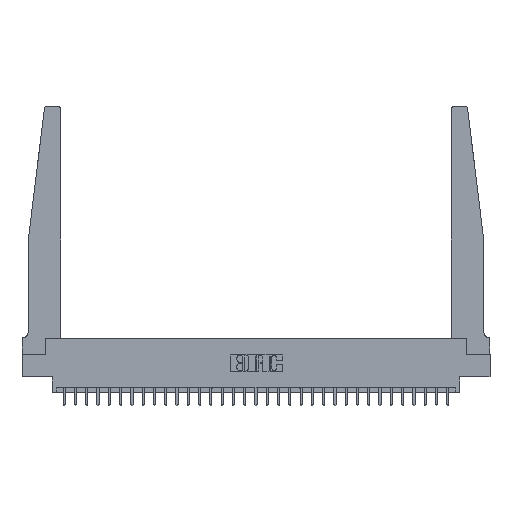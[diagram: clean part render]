
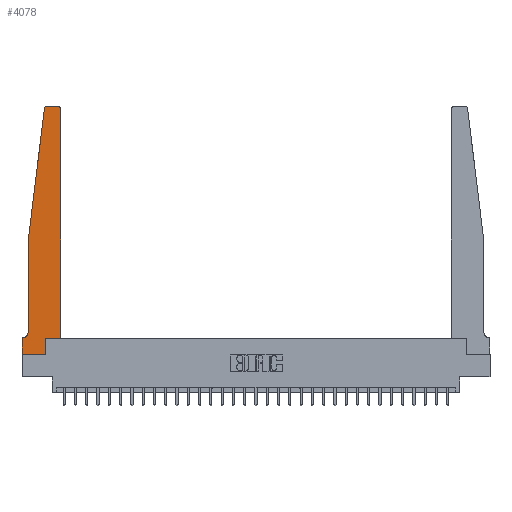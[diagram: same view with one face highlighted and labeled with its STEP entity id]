
A CAD part, top view. The second image highlights one B-rep face of the part: STEP entity #4078.
In plain terms, the highlighted planar face has unit normal (0, 0, 1).
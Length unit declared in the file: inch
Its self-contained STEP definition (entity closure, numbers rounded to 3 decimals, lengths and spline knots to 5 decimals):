
#764 = CARTESIAN_POINT ( 'NONE',  ( 0.27653, 2.75, 0.37 ) ) ;
#829 = FACE_OUTER_BOUND ( 'NONE', #19443, .T. ) ;
#895 = VERTEX_POINT ( 'NONE', #12179 ) ;
#1445 = ORIENTED_EDGE ( 'NONE', *, *, #22652, .T. ) ;
#1629 = ORIENTED_EDGE ( 'NONE', *, *, #19294, .T. ) ;
#1719 = ORIENTED_EDGE ( 'NONE', *, *, #20639, .T. ) ;
#1783 = EDGE_CURVE ( 'NONE', #9734, #4977, #10332, .T. ) ;
#1935 = CARTESIAN_POINT ( 'NONE',  ( 0.425, 2.72, 0.37 ) ) ;
#2194 = ORIENTED_EDGE ( 'NONE', *, *, #1783, .T. ) ;
#2510 = EDGE_CURVE ( 'NONE', #13632, #2628, #15795, .T. ) ;
#2628 = VERTEX_POINT ( 'NONE', #12297 ) ;
#3039 = PLANE ( 'NONE',  #23411 ) ;
#4078 = ADVANCED_FACE ( 'NONE', ( #829 ), #3039, .T. ) ;
#4294 = VERTEX_POINT ( 'NONE', #9382 ) ;
#4536 = CARTESIAN_POINT ( 'NONE',  ( 0.065, 1.25, 0.37 ) ) ;
#4634 = CARTESIAN_POINT ( 'NONE',  ( 0.425, 0.18, 0.37 ) ) ;
#4977 = VERTEX_POINT ( 'NONE', #10796 ) ;
#5024 = VECTOR ( 'NONE', #6549, 39.37008 ) ;
#5592 = VERTEX_POINT ( 'NONE', #13567 ) ;
#5667 = CARTESIAN_POINT ( 'NONE',  ( 0.425, 0.18, 0.37 ) ) ;
#6128 = LINE ( 'NONE', #6573, #9366 ) ;
#6343 = VERTEX_POINT ( 'NONE', #10515 ) ;
#6492 = LINE ( 'NONE', #9685, #26408 ) ;
#6549 = DIRECTION ( 'NONE',  ( -0.122, -0.992, 0. ) ) ;
#6573 = CARTESIAN_POINT ( 'NONE',  ( 0.065, 0.1875, 0.37 ) ) ;
#7783 = DIRECTION ( 'NONE',  ( 0., 0., 1. ) ) ;
#9280 = AXIS2_PLACEMENT_3D ( 'NONE', #16641, #12321, #14843 ) ;
#9366 = VECTOR ( 'NONE', #15596, 39.37008 ) ;
#9382 = CARTESIAN_POINT ( 'NONE',  ( 0.395, 2.75, 0.37 ) ) ;
#9648 = DIRECTION ( 'NONE',  ( 0., 1., 0. ) ) ;
#9685 = CARTESIAN_POINT ( 'NONE',  ( 0., 0., 0.37 ) ) ;
#9734 = VERTEX_POINT ( 'NONE', #24528 ) ;
#10059 = VECTOR ( 'NONE', #18448, 39.37008 ) ;
#10228 = ORIENTED_EDGE ( 'NONE', *, *, #18574, .T. ) ;
#10332 = LINE ( 'NONE', #20980, #11609 ) ;
#10515 = CARTESIAN_POINT ( 'NONE',  ( 0., 0.1875, 0.37 ) ) ;
#10796 = CARTESIAN_POINT ( 'NONE',  ( 0.2605, 0.18, 0.37 ) ) ;
#10844 = DIRECTION ( 'NONE',  ( 0., 0., -1. ) ) ;
#11584 = VECTOR ( 'NONE', #13251, 39.37008 ) ;
#11609 = VECTOR ( 'NONE', #14493, 39.37008 ) ;
#11685 = ORIENTED_EDGE ( 'NONE', *, *, #26746, .T. ) ;
#12131 = EDGE_CURVE ( 'NONE', #2628, #895, #24885, .T. ) ;
#12179 = CARTESIAN_POINT ( 'NONE',  ( 0.015, 0.1875, 0.37 ) ) ;
#12297 = CARTESIAN_POINT ( 'NONE',  ( 0.065, 0.2375, 0.37 ) ) ;
#12321 = DIRECTION ( 'NONE',  ( 0., 0., 1. ) ) ;
#12524 = DIRECTION ( 'NONE',  ( 0., 0., 1. ) ) ;
#12640 = VERTEX_POINT ( 'NONE', #1935 ) ;
#13251 = DIRECTION ( 'NONE',  ( -1., 0., 0. ) ) ;
#13420 = ORIENTED_EDGE ( 'NONE', *, *, #2510, .T. ) ;
#13567 = CARTESIAN_POINT ( 'NONE',  ( 0., 0., 0.37 ) ) ;
#13612 = ORIENTED_EDGE ( 'NONE', *, *, #20744, .T. ) ;
#13632 = VERTEX_POINT ( 'NONE', #26166 ) ;
#13639 = CARTESIAN_POINT ( 'NONE',  ( 0., 0., 0.37 ) ) ;
#13667 = LINE ( 'NONE', #4634, #24082 ) ;
#14493 = DIRECTION ( 'NONE',  ( 0., 1., 0. ) ) ;
#14835 = DIRECTION ( 'NONE',  ( 1., 0., 0. ) ) ;
#14843 = DIRECTION ( 'NONE',  ( 1., 0., 0. ) ) ;
#14905 = CARTESIAN_POINT ( 'NONE',  ( 0.27653, 2.72, 0.37 ) ) ;
#15496 = CARTESIAN_POINT ( 'NONE',  ( 0.25, 2.75, 0.37 ) ) ;
#15596 = DIRECTION ( 'NONE',  ( -1., 0., 0. ) ) ;
#15706 = EDGE_CURVE ( 'NONE', #6343, #5592, #17655, .T. ) ;
#15795 = LINE ( 'NONE', #4536, #10059 ) ;
#16641 = CARTESIAN_POINT ( 'NONE',  ( 0.395, 2.72, 0.37 ) ) ;
#16959 = AXIS2_PLACEMENT_3D ( 'NONE', #14905, #12524, #19343 ) ;
#16987 = ORIENTED_EDGE ( 'NONE', *, *, #23023, .T. ) ;
#17655 = LINE ( 'NONE', #13639, #22836 ) ;
#18322 = AXIS2_PLACEMENT_3D ( 'NONE', #19724, #10844, #21916 ) ;
#18448 = DIRECTION ( 'NONE',  ( 0., -1., 0. ) ) ;
#18574 = EDGE_CURVE ( 'NONE', #4294, #22357, #19912, .T. ) ;
#18887 = DIRECTION ( 'NONE',  ( 1., 0., 0. ) ) ;
#18910 = ORIENTED_EDGE ( 'NONE', *, *, #15706, .T. ) ;
#19155 = VECTOR ( 'NONE', #14835, 39.37008 ) ;
#19294 = EDGE_CURVE ( 'NONE', #4977, #27153, #21480, .T. ) ;
#19343 = DIRECTION ( 'NONE',  ( 1., 0., 0. ) ) ;
#19443 = EDGE_LOOP ( 'NONE', ( #10228, #1445, #13612, #13420, #23301, #16987, #18910, #11685, #2194, #1629, #28162, #1719 ) ) ;
#19724 = CARTESIAN_POINT ( 'NONE',  ( 0.015, 0.2375, 0.37 ) ) ;
#19912 = LINE ( 'NONE', #15496, #11584 ) ;
#20639 = EDGE_CURVE ( 'NONE', #12640, #4294, #23877, .T. ) ;
#20744 = EDGE_CURVE ( 'NONE', #26954, #13632, #21901, .T. ) ;
#20980 = CARTESIAN_POINT ( 'NONE',  ( 0.2605, 0.18, 0.37 ) ) ;
#21480 = LINE ( 'NONE', #5667, #19155 ) ;
#21901 = LINE ( 'NONE', #28800, #5024 ) ;
#21916 = DIRECTION ( 'NONE',  ( -1., 0., 0. ) ) ;
#22357 = VERTEX_POINT ( 'NONE', #764 ) ;
#22627 = DIRECTION ( 'NONE',  ( 0., -1., 0. ) ) ;
#22652 = EDGE_CURVE ( 'NONE', #22357, #26954, #28653, .T. ) ;
#22832 = DIRECTION ( 'NONE',  ( 1., 0., 0. ) ) ;
#22836 = VECTOR ( 'NONE', #22627, 39.37008 ) ;
#23023 = EDGE_CURVE ( 'NONE', #895, #6343, #6128, .T. ) ;
#23115 = EDGE_CURVE ( 'NONE', #27153, #12640, #13667, .T. ) ;
#23301 = ORIENTED_EDGE ( 'NONE', *, *, #12131, .T. ) ;
#23325 = CARTESIAN_POINT ( 'NONE',  ( 0.24675, 2.72367, 0.37 ) ) ;
#23411 = AXIS2_PLACEMENT_3D ( 'NONE', #25498, #7783, #18887 ) ;
#23877 = CIRCLE ( 'NONE', #9280, 0.03 ) ;
#24082 = VECTOR ( 'NONE', #9648, 39.37008 ) ;
#24528 = CARTESIAN_POINT ( 'NONE',  ( 0.2605, 0., 0.37 ) ) ;
#24885 = CIRCLE ( 'NONE', #18322, 0.05 ) ;
#24932 = CARTESIAN_POINT ( 'NONE',  ( 0.425, 0.18, 0.37 ) ) ;
#25498 = CARTESIAN_POINT ( 'NONE',  ( 0., 0.1875, 0.37 ) ) ;
#26166 = CARTESIAN_POINT ( 'NONE',  ( 0.065, 1.25, 0.37 ) ) ;
#26408 = VECTOR ( 'NONE', #22832, 39.37008 ) ;
#26746 = EDGE_CURVE ( 'NONE', #5592, #9734, #6492, .T. ) ;
#26954 = VERTEX_POINT ( 'NONE', #23325 ) ;
#27153 = VERTEX_POINT ( 'NONE', #24932 ) ;
#28162 = ORIENTED_EDGE ( 'NONE', *, *, #23115, .T. ) ;
#28653 = CIRCLE ( 'NONE', #16959, 0.03 ) ;
#28800 = CARTESIAN_POINT ( 'NONE',  ( 0.065, 1.25, 0.37 ) ) ;
